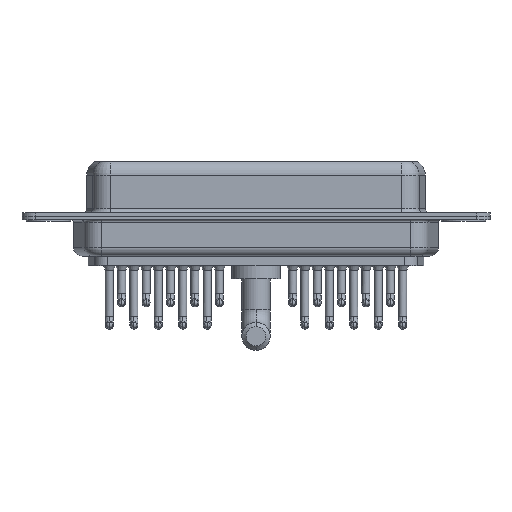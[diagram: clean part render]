
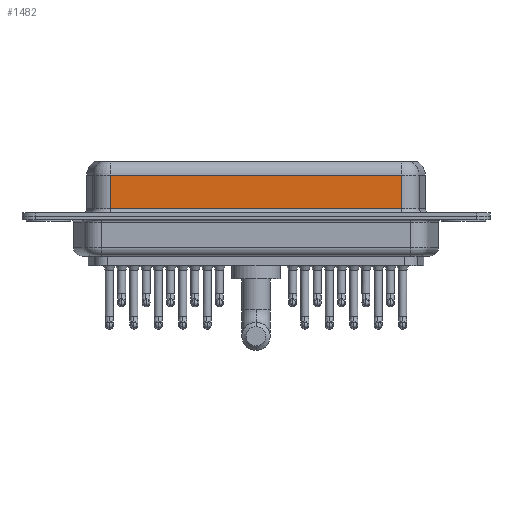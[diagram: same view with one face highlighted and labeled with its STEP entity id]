
A CAD part, front view. The second image highlights one B-rep face of the part: STEP entity #1482.
In plain terms, the highlighted planar face has unit normal (0, -1, 0).
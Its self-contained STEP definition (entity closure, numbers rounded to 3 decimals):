
#30 = CARTESIAN_POINT ( 'NONE',  ( 7.013, -3.95, 0.9 ) ) ;
#188 = FACE_OUTER_BOUND ( 'NONE', #7097, .T. ) ;
#328 = LINE ( 'NONE', #2129, #16086 ) ;
#342 = DIRECTION ( 'NONE',  ( 0., 0., -1. ) ) ;
#940 = EDGE_CURVE ( 'NONE', #11126, #6649, #328, .T. ) ;
#1482 = ADVANCED_FACE ( 'NONE', ( #188 ), #12942, .F. ) ;
#1762 = CARTESIAN_POINT ( 'NONE',  ( 40.037, -3.95, 6.4 ) ) ;
#1809 = DIRECTION ( 'NONE',  ( 1., 0., 0. ) ) ;
#2129 = CARTESIAN_POINT ( 'NONE',  ( 40.037, -3.95, 0.9 ) ) ;
#3181 = CARTESIAN_POINT ( 'NONE',  ( 40.037, -3.95, 6.4 ) ) ;
#3191 = CARTESIAN_POINT ( 'NONE',  ( 7.013, -3.95, 6.4 ) ) ;
#4319 = VECTOR ( 'NONE', #8964, 1000. ) ;
#4814 = DIRECTION ( 'NONE',  ( 0., 1., 0. ) ) ;
#5204 = ORIENTED_EDGE ( 'NONE', *, *, #940, .T. ) ;
#6169 = VERTEX_POINT ( 'NONE', #17245 ) ;
#6649 = VERTEX_POINT ( 'NONE', #15848 ) ;
#7097 = EDGE_LOOP ( 'NONE', ( #18497, #17880, #11905, #5204 ) ) ;
#8964 = DIRECTION ( 'NONE',  ( -1., 0., 0. ) ) ;
#9610 = DIRECTION ( 'NONE',  ( 0., 0., -1. ) ) ;
#10220 = VECTOR ( 'NONE', #342, 1000. ) ;
#10534 = LINE ( 'NONE', #20160, #4319 ) ;
#11126 = VERTEX_POINT ( 'NONE', #30 ) ;
#11905 = ORIENTED_EDGE ( 'NONE', *, *, #13042, .T. ) ;
#12469 = CARTESIAN_POINT ( 'NONE',  ( 7.013, -3.95, 4.65 ) ) ;
#12942 = PLANE ( 'NONE',  #20221 ) ;
#13042 = EDGE_CURVE ( 'NONE', #17368, #11126, #19644, .T. ) ;
#15620 = EDGE_CURVE ( 'NONE', #6169, #17368, #10534, .T. ) ;
#15848 = CARTESIAN_POINT ( 'NONE',  ( 40.037, -3.95, 0.9 ) ) ;
#15926 = VECTOR ( 'NONE', #9610, 1000. ) ;
#16086 = VECTOR ( 'NONE', #1809, 1000. ) ;
#17245 = CARTESIAN_POINT ( 'NONE',  ( 40.037, -3.95, 4.65 ) ) ;
#17368 = VERTEX_POINT ( 'NONE', #12469 ) ;
#17382 = DIRECTION ( 'NONE',  ( 0., 0., 1. ) ) ;
#17642 = LINE ( 'NONE', #3181, #15926 ) ;
#17880 = ORIENTED_EDGE ( 'NONE', *, *, #15620, .T. ) ;
#18483 = EDGE_CURVE ( 'NONE', #6169, #6649, #17642, .T. ) ;
#18497 = ORIENTED_EDGE ( 'NONE', *, *, #18483, .F. ) ;
#19644 = LINE ( 'NONE', #3191, #10220 ) ;
#20160 = CARTESIAN_POINT ( 'NONE',  ( 40.037, -3.95, 4.65 ) ) ;
#20221 = AXIS2_PLACEMENT_3D ( 'NONE', #1762, #4814, #17382 ) ;
